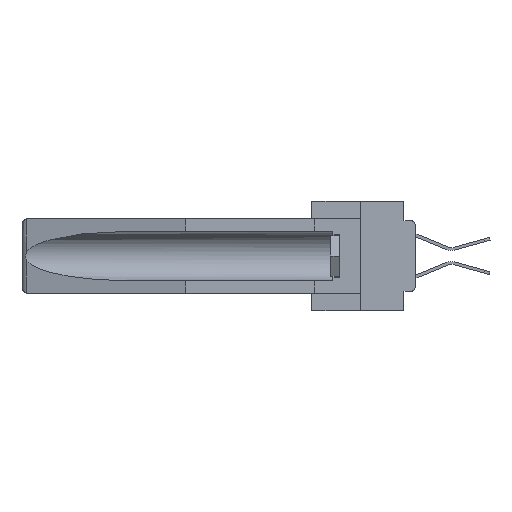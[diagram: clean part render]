
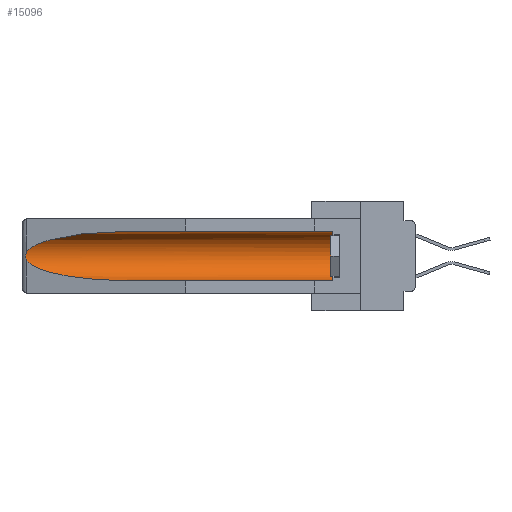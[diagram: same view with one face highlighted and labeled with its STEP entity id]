
A CAD part, left-side view. The second image highlights one B-rep face of the part: STEP entity #15096.
In plain terms, the highlighted cylindrical face has radius 2.857 mm (diameter 5.715 mm), a partial arc.
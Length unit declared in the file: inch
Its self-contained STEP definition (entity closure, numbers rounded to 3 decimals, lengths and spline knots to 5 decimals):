
#17 = DIRECTION ( 'NONE',  ( 0., 0., 1. ) ) ;
#1479 = CARTESIAN_POINT ( 'NONE',  ( 0.26597, 1.52961, -0.15275 ) ) ;
#2213 = ORIENTED_EDGE ( 'NONE', *, *, #16686, .T. ) ;
#2247 =( BOUNDED_CURVE ( )  B_SPLINE_CURVE ( 3, ( #17977, #4829, #15153, #2448 ),
 .UNSPECIFIED., .F., .F. ) 
 B_SPLINE_CURVE_WITH_KNOTS ( ( 4, 4 ),
 ( 0.1948, 1.5708 ),
 .UNSPECIFIED. ) 
 CURVE ( )  GEOMETRIC_REPRESENTATION_ITEM ( )  RATIONAL_B_SPLINE_CURVE ( ( 1., 0.848, 0.848, 1. ) ) 
 REPRESENTATION_ITEM ( '' )  );
#2307 = CARTESIAN_POINT ( 'NONE',  ( 0.21114, 1.30732, -0.059 ) ) ;
#2448 = CARTESIAN_POINT ( 'NONE',  ( 0.155, 1.07973, -0.284 ) ) ;
#2471 = EDGE_CURVE ( 'NONE', #10523, #18739, #14346, .T. ) ;
#2895 = CARTESIAN_POINT ( 'NONE',  ( 0.155, 0.126, -0.059 ) ) ;
#3976 = CARTESIAN_POINT ( 'NONE',  ( 0.26537, 1.52718, -0.14972 ) ) ;
#4088 = CARTESIAN_POINT ( 'NONE',  ( 0.2675, 1.53308, -0.17534 ) ) ;
#4829 = CARTESIAN_POINT ( 'NONE',  ( 0.25451, 1.48313, -0.24835 ) ) ;
#5053 = CARTESIAN_POINT ( 'NONE',  ( 0.155, 1.07973, -0.284 ) ) ;
#5581 = AXIS2_PLACEMENT_3D ( 'NONE', #6223, #24043, #21757 ) ;
#6223 = CARTESIAN_POINT ( 'NONE',  ( 0.155, 0.126, -0.1715 ) ) ;
#6224 = VERTEX_POINT ( 'NONE', #8574 ) ;
#6614 = CARTESIAN_POINT ( 'NONE',  ( 0.2673, 1.5327, -0.16383 ) ) ;
#7313 = ORIENTED_EDGE ( 'NONE', *, *, #23307, .T. ) ;
#7560 = CARTESIAN_POINT ( 'NONE',  ( 0.155, 1.07973, -0.059 ) ) ;
#7784 = CARTESIAN_POINT ( 'NONE',  ( 0.26537, 1.52718, -0.14972 ) ) ;
#8574 = CARTESIAN_POINT ( 'NONE',  ( 0.26537, 1.52718, -0.19328 ) ) ;
#9116 = CARTESIAN_POINT ( 'NONE',  ( 0.2673, 1.53269, -0.17917 ) ) ;
#9464 = CARTESIAN_POINT ( 'NONE',  ( 0.26537, 1.52718, -0.19328 ) ) ;
#9466 = EDGE_CURVE ( 'NONE', #10523, #29709, #32136, .T. ) ;
#9548 = CYLINDRICAL_SURFACE ( 'NONE', #26703, 0.1125 ) ;
#9710 = EDGE_LOOP ( 'NONE', ( #29718, #19252, #7313, #21281, #10965, #2213 ) ) ;
#10523 = VERTEX_POINT ( 'NONE', #10806 ) ;
#10633 = CARTESIAN_POINT ( 'NONE',  ( 0.155, -0.30754, -0.284 ) ) ;
#10806 = CARTESIAN_POINT ( 'NONE',  ( 0.155, 0.126, -0.284 ) ) ;
#10965 = ORIENTED_EDGE ( 'NONE', *, *, #9466, .T. ) ;
#11595 = EDGE_CURVE ( 'NONE', #32053, #6224, #23579, .T. ) ;
#12002 = CARTESIAN_POINT ( 'NONE',  ( 0.26654, 1.53092, -0.15636 ) ) ;
#12058 = CARTESIAN_POINT ( 'NONE',  ( 0.155, -0.30754, -0.059 ) ) ;
#14346 = LINE ( 'NONE', #10633, #26993 ) ;
#15039 = EDGE_CURVE ( 'NONE', #24925, #32053, #19569, .T. ) ;
#15096 = ADVANCED_FACE ( 'NONE', ( #17737 ), #9548, .F. ) ;
#15153 = CARTESIAN_POINT ( 'NONE',  ( 0.21114, 1.30732, -0.284 ) ) ;
#16686 = EDGE_CURVE ( 'NONE', #29709, #24925, #26245, .T. ) ;
#17371 = CARTESIAN_POINT ( 'NONE',  ( 0.26655, 1.53094, -0.18657 ) ) ;
#17737 = FACE_OUTER_BOUND ( 'NONE', #9710, .T. ) ;
#17977 = CARTESIAN_POINT ( 'NONE',  ( 0.26537, 1.52718, -0.19328 ) ) ;
#18739 = VERTEX_POINT ( 'NONE', #5053 ) ;
#19252 = ORIENTED_EDGE ( 'NONE', *, *, #11595, .T. ) ;
#19257 = VECTOR ( 'NONE', #27776, 39.37008 ) ;
#19569 =( BOUNDED_CURVE ( )  B_SPLINE_CURVE ( 3, ( #7560, #2307, #33553, #7784 ),
 .UNSPECIFIED., .F., .T. ) 
 B_SPLINE_CURVE_WITH_KNOTS ( ( 4, 4 ),
 ( 4.71239, 6.08839 ),
 .UNSPECIFIED. ) 
 CURVE ( )  GEOMETRIC_REPRESENTATION_ITEM ( )  RATIONAL_B_SPLINE_CURVE ( ( 1., 0.848, 0.848, 1. ) ) 
 REPRESENTATION_ITEM ( '' )  );
#21281 = ORIENTED_EDGE ( 'NONE', *, *, #2471, .F. ) ;
#21757 = DIRECTION ( 'NONE',  ( 0., 0., 1. ) ) ;
#23307 = EDGE_CURVE ( 'NONE', #6224, #18739, #2247, .T. ) ;
#23579 = B_SPLINE_CURVE_WITH_KNOTS ( 'NONE', 3,
 ( #3976, #1479, #12002, #6614, #32959, #4088, #9116, #17371, #27490, #9464 ),
 .UNSPECIFIED., .F., .F.,
 ( 4, 2, 2, 2, 4 ),
 ( 0., 0.00029, 0.00058, 0.00087, 0.00117 ),
 .UNSPECIFIED. ) ;
#23911 = CARTESIAN_POINT ( 'NONE',  ( 0.26537, 1.52718, -0.14972 ) ) ;
#24043 = DIRECTION ( 'NONE',  ( 0., -1., 0. ) ) ;
#24925 = VERTEX_POINT ( 'NONE', #25048 ) ;
#25048 = CARTESIAN_POINT ( 'NONE',  ( 0.155, 1.07973, -0.059 ) ) ;
#26245 = LINE ( 'NONE', #12058, #19257 ) ;
#26703 = AXIS2_PLACEMENT_3D ( 'NONE', #33673, #28547, #17 ) ;
#26993 = VECTOR ( 'NONE', #28991, 39.37008 ) ;
#27490 = CARTESIAN_POINT ( 'NONE',  ( 0.26597, 1.5296, -0.19026 ) ) ;
#27776 = DIRECTION ( 'NONE',  ( 0., 1., 0. ) ) ;
#28547 = DIRECTION ( 'NONE',  ( 0., 1., 0. ) ) ;
#28991 = DIRECTION ( 'NONE',  ( 0., 1., 0. ) ) ;
#29709 = VERTEX_POINT ( 'NONE', #2895 ) ;
#29718 = ORIENTED_EDGE ( 'NONE', *, *, #15039, .T. ) ;
#32053 = VERTEX_POINT ( 'NONE', #23911 ) ;
#32136 = CIRCLE ( 'NONE', #5581, 0.1125 ) ;
#32959 = CARTESIAN_POINT ( 'NONE',  ( 0.2675, 1.53308, -0.16763 ) ) ;
#33553 = CARTESIAN_POINT ( 'NONE',  ( 0.25451, 1.48313, -0.09465 ) ) ;
#33673 = CARTESIAN_POINT ( 'NONE',  ( 0.155, -0.30754, -0.1715 ) ) ;
